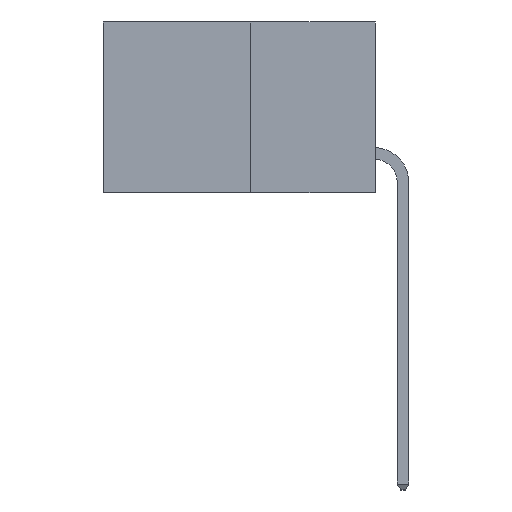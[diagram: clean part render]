
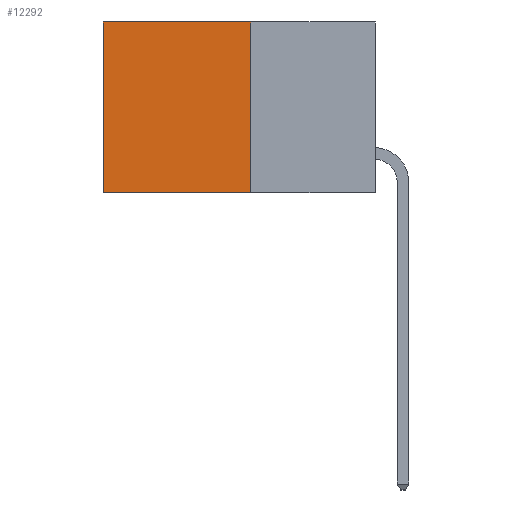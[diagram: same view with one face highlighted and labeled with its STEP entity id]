
A CAD part, left-side view. The second image highlights one B-rep face of the part: STEP entity #12292.
In plain terms, the highlighted planar face has unit normal (-1, 0, 0).
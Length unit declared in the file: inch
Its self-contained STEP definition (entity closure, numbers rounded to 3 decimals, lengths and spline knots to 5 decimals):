
#290 = VERTEX_POINT ( 'NONE', #12171 ) ;
#367 = VERTEX_POINT ( 'NONE', #3781 ) ;
#623 = VECTOR ( 'NONE', #6147, 39.37008 ) ;
#1943 = EDGE_CURVE ( 'NONE', #6216, #290, #9195, .T. ) ;
#2710 = CARTESIAN_POINT ( 'NONE',  ( 0.277, 0.59, -0.37 ) ) ;
#3781 = CARTESIAN_POINT ( 'NONE',  ( 0.277, 0.27, 0. ) ) ;
#3985 = VECTOR ( 'NONE', #12217, 39.37008 ) ;
#4150 = EDGE_CURVE ( 'NONE', #367, #6216, #11345, .T. ) ;
#4535 = EDGE_LOOP ( 'NONE', ( #9340, #11841, #8626, #9805 ) ) ;
#4625 = EDGE_CURVE ( 'NONE', #367, #8609, #5952, .T. ) ;
#4745 = CARTESIAN_POINT ( 'NONE',  ( 0.277, 0.59, 0. ) ) ;
#4999 = CARTESIAN_POINT ( 'NONE',  ( 0.277, 0.27, -0.37 ) ) ;
#5032 = CARTESIAN_POINT ( 'NONE',  ( 0.277, 0.27, 0. ) ) ;
#5112 = PLANE ( 'NONE',  #5719 ) ;
#5719 = AXIS2_PLACEMENT_3D ( 'NONE', #8039, #11819, #6105 ) ;
#5952 = LINE ( 'NONE', #5032, #623 ) ;
#6105 = DIRECTION ( 'NONE',  ( 0., 0., -1. ) ) ;
#6147 = DIRECTION ( 'NONE',  ( 0., 1., 0. ) ) ;
#6216 = VERTEX_POINT ( 'NONE', #4999 ) ;
#8039 = CARTESIAN_POINT ( 'NONE',  ( 0.277, 0.27, -0.37 ) ) ;
#8609 = VERTEX_POINT ( 'NONE', #4745 ) ;
#8626 = ORIENTED_EDGE ( 'NONE', *, *, #4150, .F. ) ;
#8854 = VECTOR ( 'NONE', #11032, 39.37008 ) ;
#9195 = LINE ( 'NONE', #11820, #3985 ) ;
#9338 = VECTOR ( 'NONE', #10500, 39.37008 ) ;
#9340 = ORIENTED_EDGE ( 'NONE', *, *, #10254, .T. ) ;
#9805 = ORIENTED_EDGE ( 'NONE', *, *, #4625, .T. ) ;
#10178 = FACE_OUTER_BOUND ( 'NONE', #4535, .T. ) ;
#10254 = EDGE_CURVE ( 'NONE', #8609, #290, #11839, .T. ) ;
#10500 = DIRECTION ( 'NONE',  ( 0., 0., -1. ) ) ;
#10998 = CARTESIAN_POINT ( 'NONE',  ( 0.277, 0.27, -0.37 ) ) ;
#11032 = DIRECTION ( 'NONE',  ( 0., 0., -1. ) ) ;
#11345 = LINE ( 'NONE', #10998, #8854 ) ;
#11819 = DIRECTION ( 'NONE',  ( 1., 0., 0. ) ) ;
#11820 = CARTESIAN_POINT ( 'NONE',  ( 0.277, 0.27, -0.37 ) ) ;
#11839 = LINE ( 'NONE', #2710, #9338 ) ;
#11841 = ORIENTED_EDGE ( 'NONE', *, *, #1943, .F. ) ;
#12171 = CARTESIAN_POINT ( 'NONE',  ( 0.277, 0.59, -0.37 ) ) ;
#12217 = DIRECTION ( 'NONE',  ( 0., 1., 0. ) ) ;
#12292 = ADVANCED_FACE ( 'NONE', ( #10178 ), #5112, .F. ) ;
